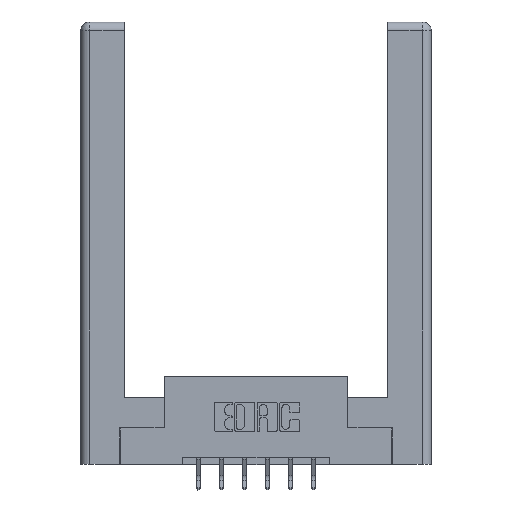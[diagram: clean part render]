
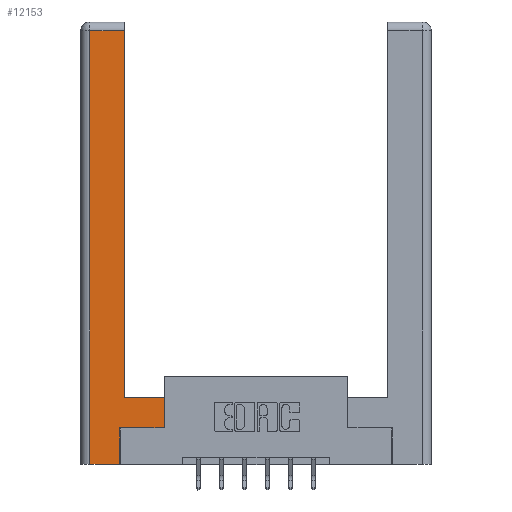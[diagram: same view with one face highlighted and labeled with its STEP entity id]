
A CAD part, top view. The second image highlights one B-rep face of the part: STEP entity #12153.
In plain terms, the highlighted planar face has unit normal (0, 0, 1).
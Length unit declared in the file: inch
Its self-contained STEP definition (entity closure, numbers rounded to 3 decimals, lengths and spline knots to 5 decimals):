
#36 = FACE_OUTER_BOUND ( 'NONE', #4489, .T. ) ;
#186 = CARTESIAN_POINT ( 'NONE',  ( 0.265, 0., 0. ) ) ;
#389 = LINE ( 'NONE', #1370, #10090 ) ;
#577 = ORIENTED_EDGE ( 'NONE', *, *, #12112, .T. ) ;
#708 = CARTESIAN_POINT ( 'NONE',  ( 0.295, 0.45, 0. ) ) ;
#889 = ORIENTED_EDGE ( 'NONE', *, *, #10315, .T. ) ;
#1145 = LINE ( 'NONE', #6235, #7009 ) ;
#1370 = CARTESIAN_POINT ( 'NONE',  ( 0.565, 0.245, 0. ) ) ;
#1516 = CARTESIAN_POINT ( 'NONE',  ( 0.295, 2.94, 0. ) ) ;
#1576 = DIRECTION ( 'NONE',  ( 0., 1., 0. ) ) ;
#1589 = LINE ( 'NONE', #3258, #10997 ) ;
#1743 = CARTESIAN_POINT ( 'NONE',  ( 0.565, 0.245, 0. ) ) ;
#2004 = EDGE_CURVE ( 'NONE', #6098, #7404, #3125, .T. ) ;
#2467 = ORIENTED_EDGE ( 'NONE', *, *, #8334, .T. ) ;
#2696 = VERTEX_POINT ( 'NONE', #9497 ) ;
#3125 = LINE ( 'NONE', #3311, #9749 ) ;
#3228 = VERTEX_POINT ( 'NONE', #9508 ) ;
#3258 = CARTESIAN_POINT ( 'NONE',  ( 0.265, 0., 0. ) ) ;
#3311 = CARTESIAN_POINT ( 'NONE',  ( 0.295, 3., 0. ) ) ;
#3465 = DIRECTION ( 'NONE',  ( 0., -1., 0. ) ) ;
#3557 = VERTEX_POINT ( 'NONE', #1743 ) ;
#3836 = EDGE_CURVE ( 'NONE', #3557, #9654, #8980, .T. ) ;
#4030 = EDGE_CURVE ( 'NONE', #9654, #6098, #6172, .T. ) ;
#4213 = ORIENTED_EDGE ( 'NONE', *, *, #4405, .T. ) ;
#4400 = CARTESIAN_POINT ( 'NONE',  ( 0.565, 0.45, 0. ) ) ;
#4405 = EDGE_CURVE ( 'NONE', #7404, #7164, #6306, .T. ) ;
#4489 = EDGE_LOOP ( 'NONE', ( #6632, #4213, #889, #2467, #577, #7030, #12079, #9524 ) ) ;
#4730 = AXIS2_PLACEMENT_3D ( 'NONE', #5392, #5311, #6226 ) ;
#5005 = CARTESIAN_POINT ( 'NONE',  ( 0.565, 0.45, 0. ) ) ;
#5264 = DIRECTION ( 'NONE',  ( -1., 0., 0. ) ) ;
#5286 = VECTOR ( 'NONE', #10727, 39.37008 ) ;
#5311 = DIRECTION ( 'NONE',  ( 0., 0., -1. ) ) ;
#5392 = CARTESIAN_POINT ( 'NONE',  ( 0., 0., 0. ) ) ;
#5838 = VERTEX_POINT ( 'NONE', #186 ) ;
#5874 = CARTESIAN_POINT ( 'NONE',  ( 0.0615, 2.94, 0. ) ) ;
#6075 = VECTOR ( 'NONE', #11967, 39.37008 ) ;
#6098 = VERTEX_POINT ( 'NONE', #708 ) ;
#6172 = LINE ( 'NONE', #8485, #10141 ) ;
#6226 = DIRECTION ( 'NONE',  ( -1., 0., 0. ) ) ;
#6235 = CARTESIAN_POINT ( 'NONE',  ( 0.0615, 0., 0. ) ) ;
#6306 = LINE ( 'NONE', #9869, #7926 ) ;
#6395 = CARTESIAN_POINT ( 'NONE',  ( 0.265, 0.245, 0. ) ) ;
#6561 = EDGE_CURVE ( 'NONE', #3228, #3557, #389, .T. ) ;
#6632 = ORIENTED_EDGE ( 'NONE', *, *, #2004, .T. ) ;
#7009 = VECTOR ( 'NONE', #3465, 39.37008 ) ;
#7030 = ORIENTED_EDGE ( 'NONE', *, *, #6561, .T. ) ;
#7164 = VERTEX_POINT ( 'NONE', #5874 ) ;
#7293 = PLANE ( 'NONE',  #4730 ) ;
#7404 = VERTEX_POINT ( 'NONE', #1516 ) ;
#7926 = VECTOR ( 'NONE', #5264, 39.37008 ) ;
#8334 = EDGE_CURVE ( 'NONE', #2696, #5838, #1589, .T. ) ;
#8485 = CARTESIAN_POINT ( 'NONE',  ( 0.295, 0.45, 0. ) ) ;
#8724 = DIRECTION ( 'NONE',  ( 1., 0., 0. ) ) ;
#8980 = LINE ( 'NONE', #5005, #5286 ) ;
#9497 = CARTESIAN_POINT ( 'NONE',  ( 0.0615, 0., 0. ) ) ;
#9508 = CARTESIAN_POINT ( 'NONE',  ( 0.265, 0.245, 0. ) ) ;
#9524 = ORIENTED_EDGE ( 'NONE', *, *, #4030, .T. ) ;
#9654 = VERTEX_POINT ( 'NONE', #4400 ) ;
#9749 = VECTOR ( 'NONE', #1576, 39.37008 ) ;
#9869 = CARTESIAN_POINT ( 'NONE',  ( 0.0615, 2.94, 0. ) ) ;
#9887 = LINE ( 'NONE', #6395, #6075 ) ;
#9894 = DIRECTION ( 'NONE',  ( 1., 0., 0. ) ) ;
#10090 = VECTOR ( 'NONE', #8724, 39.37008 ) ;
#10141 = VECTOR ( 'NONE', #10375, 39.37008 ) ;
#10315 = EDGE_CURVE ( 'NONE', #7164, #2696, #1145, .T. ) ;
#10375 = DIRECTION ( 'NONE',  ( -1., 0., 0. ) ) ;
#10727 = DIRECTION ( 'NONE',  ( 0., 1., 0. ) ) ;
#10997 = VECTOR ( 'NONE', #9894, 39.37008 ) ;
#11967 = DIRECTION ( 'NONE',  ( 0., 1., 0. ) ) ;
#12079 = ORIENTED_EDGE ( 'NONE', *, *, #3836, .T. ) ;
#12112 = EDGE_CURVE ( 'NONE', #5838, #3228, #9887, .T. ) ;
#12153 = ADVANCED_FACE ( 'NONE', ( #36 ), #7293, .F. ) ;
